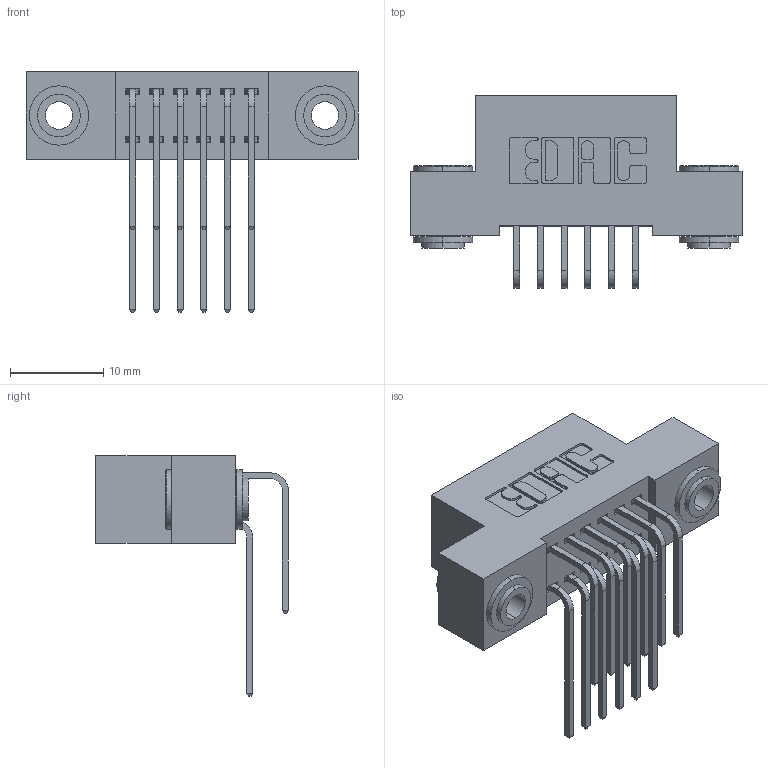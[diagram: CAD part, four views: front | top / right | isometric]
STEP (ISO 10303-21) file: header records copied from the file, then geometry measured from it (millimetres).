
FILE_DESCRIPTION (( 'STEP AP203' ), '1' );
FILE_NAME ('392-012-559-203.STEP', '2019-10-07T01:44:06', ( '' ), ( '' ), 'SwSTEP 2.0', 'SolidWorks 2016', '' );
FILE_SCHEMA (( 'CONFIG_CONTROL_DESIGN' ));
Length unit declared in the file: inch
Products named in the file (5): 345-292-001_559 Tail - 2; 342-250-002_345-250-002-102; 392-012-559-203; 342 Part_.156 TH; 345-292-001_558 559 Tail - 1
Assembly tree (15 placements, depth 2):
  392-012-559-203
    342 Part_.156 TH
    345-292-001_558 559 Tail - 1  x6
    345-292-001_559 Tail - 2  x6
    342-250-002_345-250-002-102  x2
Bounding box: 35.56 x 20.64 x 25.78 mm (x, y, z)
Volume: 3116.7 mm3; surface area: 4713.4 mm2
Topology: 15 solids, 15 shells, 796 faces, 2307 edges, 1518 vertices
Faces by surface type: plane 532, cylinder 256, cone 8
Entity records: 10818 total; most frequent: CARTESIAN_POINT 1860, ORIENTED_EDGE 1738, DIRECTION 1667, EDGE_CURVE 869, VECTOR 677, LINE 677, VERTEX_POINT 574, AXIS2_PLACEMENT_3D 495
